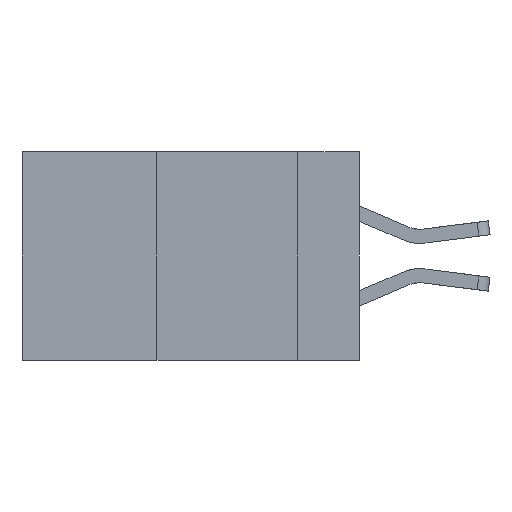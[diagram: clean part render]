
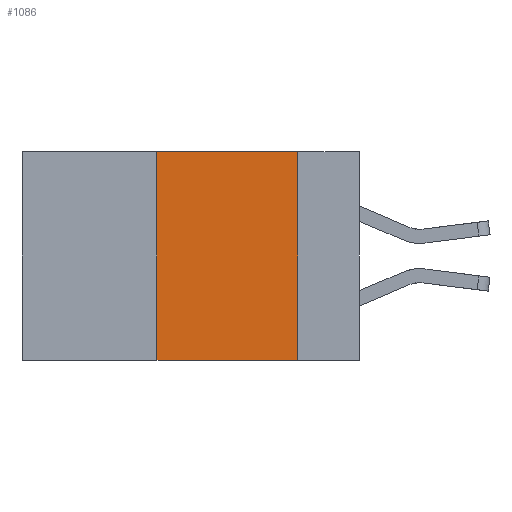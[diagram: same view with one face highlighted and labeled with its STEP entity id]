
A CAD part, left-side view. The second image highlights one B-rep face of the part: STEP entity #1086.
In plain terms, the highlighted planar face has unit normal (-1, 0, 0).
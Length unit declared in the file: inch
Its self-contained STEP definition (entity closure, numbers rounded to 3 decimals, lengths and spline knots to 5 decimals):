
#78 = EDGE_CURVE ( 'NONE', #6895, #6312, #2589, .T. ) ;
#198 = CARTESIAN_POINT ( 'NONE',  ( 0., 0.11, 0. ) ) ;
#681 = VECTOR ( 'NONE', #4744, 39.37008 ) ;
#795 = CARTESIAN_POINT ( 'NONE',  ( 0., 0.36, 0. ) ) ;
#807 = VECTOR ( 'NONE', #12151, 39.37008 ) ;
#1070 = LINE ( 'NONE', #2345, #681 ) ;
#1086 = ADVANCED_FACE ( 'NONE', ( #9115 ), #12650, .F. ) ;
#2345 = CARTESIAN_POINT ( 'NONE',  ( 0., 0.11, 0. ) ) ;
#2589 = LINE ( 'NONE', #7406, #807 ) ;
#3303 = CARTESIAN_POINT ( 'NONE',  ( 0., 0.11, -0.37 ) ) ;
#4115 = AXIS2_PLACEMENT_3D ( 'NONE', #6652, #12814, #10286 ) ;
#4744 = DIRECTION ( 'NONE',  ( 0., 0., -1. ) ) ;
#5205 = VERTEX_POINT ( 'NONE', #3303 ) ;
#5433 = DIRECTION ( 'NONE',  ( 0., -1., 0. ) ) ;
#5760 = CARTESIAN_POINT ( 'NONE',  ( 0., 0.36, -0.37 ) ) ;
#6312 = VERTEX_POINT ( 'NONE', #198 ) ;
#6650 = DIRECTION ( 'NONE',  ( 0., 0., 1. ) ) ;
#6652 = CARTESIAN_POINT ( 'NONE',  ( 0., 0.6, 0. ) ) ;
#6740 = LINE ( 'NONE', #795, #15072 ) ;
#6895 = VERTEX_POINT ( 'NONE', #10079 ) ;
#7013 = VERTEX_POINT ( 'NONE', #5760 ) ;
#7279 = EDGE_LOOP ( 'NONE', ( #13364, #11077, #10086, #14151 ) ) ;
#7406 = CARTESIAN_POINT ( 'NONE',  ( 0., 0.6, 0. ) ) ;
#8704 = VECTOR ( 'NONE', #5433, 39.37008 ) ;
#9115 = FACE_OUTER_BOUND ( 'NONE', #7279, .T. ) ;
#9949 = EDGE_CURVE ( 'NONE', #7013, #5205, #12588, .T. ) ;
#10079 = CARTESIAN_POINT ( 'NONE',  ( 0., 0.36, 0. ) ) ;
#10086 = ORIENTED_EDGE ( 'NONE', *, *, #14252, .F. ) ;
#10286 = DIRECTION ( 'NONE',  ( 0., 0., -1. ) ) ;
#11077 = ORIENTED_EDGE ( 'NONE', *, *, #78, .F. ) ;
#11406 = CARTESIAN_POINT ( 'NONE',  ( 0., 0.6, -0.37 ) ) ;
#12151 = DIRECTION ( 'NONE',  ( 0., -1., 0. ) ) ;
#12588 = LINE ( 'NONE', #11406, #8704 ) ;
#12650 = PLANE ( 'NONE',  #4115 ) ;
#12814 = DIRECTION ( 'NONE',  ( 1., 0., 0. ) ) ;
#13364 = ORIENTED_EDGE ( 'NONE', *, *, #14739, .F. ) ;
#14151 = ORIENTED_EDGE ( 'NONE', *, *, #9949, .T. ) ;
#14252 = EDGE_CURVE ( 'NONE', #7013, #6895, #6740, .T. ) ;
#14739 = EDGE_CURVE ( 'NONE', #6312, #5205, #1070, .T. ) ;
#15072 = VECTOR ( 'NONE', #6650, 39.37008 ) ;
